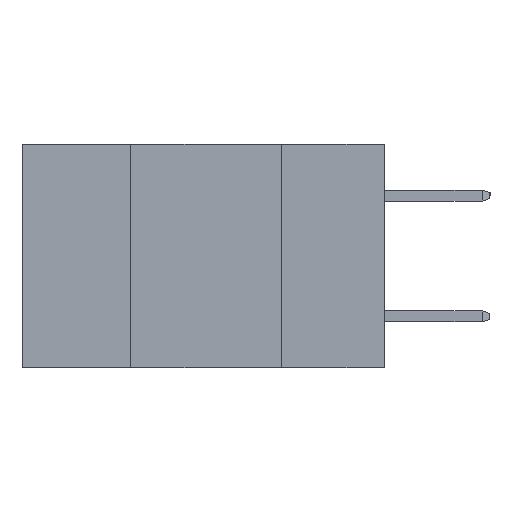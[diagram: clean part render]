
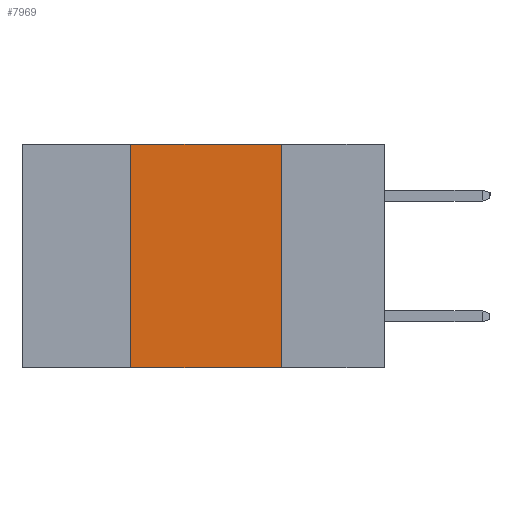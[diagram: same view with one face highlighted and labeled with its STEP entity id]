
A CAD part, left-side view. The second image highlights one B-rep face of the part: STEP entity #7969.
In plain terms, the highlighted planar face has unit normal (-1, 0, 0).
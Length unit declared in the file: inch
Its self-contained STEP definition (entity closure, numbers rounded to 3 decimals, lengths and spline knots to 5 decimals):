
#943 = DIRECTION ( 'NONE',  ( 0., 0., 1. ) ) ;
#1588 = VERTEX_POINT ( 'NONE', #14221 ) ;
#1596 = CARTESIAN_POINT ( 'NONE',  ( 0., 0.6, 0. ) ) ;
#1762 = PLANE ( 'NONE',  #10944 ) ;
#1893 = VECTOR ( 'NONE', #6723, 39.37008 ) ;
#2411 = VECTOR ( 'NONE', #6153, 39.37008 ) ;
#2767 = EDGE_LOOP ( 'NONE', ( #6430, #9768, #9889, #12947 ) ) ;
#2978 = VERTEX_POINT ( 'NONE', #11279 ) ;
#3924 = DIRECTION ( 'NONE',  ( 1., 0., 0. ) ) ;
#4325 = LINE ( 'NONE', #9272, #7523 ) ;
#4781 = CARTESIAN_POINT ( 'NONE',  ( 0., 0.42, -0.37 ) ) ;
#5536 = DIRECTION ( 'NONE',  ( 0., -1., 0. ) ) ;
#6153 = DIRECTION ( 'NONE',  ( 0., -1., 0. ) ) ;
#6430 = ORIENTED_EDGE ( 'NONE', *, *, #9613, .F. ) ;
#6723 = DIRECTION ( 'NONE',  ( 0., 0., -1. ) ) ;
#7523 = VECTOR ( 'NONE', #5536, 39.37008 ) ;
#7969 = ADVANCED_FACE ( 'NONE', ( #9104 ), #1762, .F. ) ;
#8082 = CARTESIAN_POINT ( 'NONE',  ( 0., 0.17, -0.37 ) ) ;
#8877 = DIRECTION ( 'NONE',  ( 0., 0., -1. ) ) ;
#9104 = FACE_OUTER_BOUND ( 'NONE', #2767, .T. ) ;
#9272 = CARTESIAN_POINT ( 'NONE',  ( 0., 0.6, -0.37 ) ) ;
#9613 = EDGE_CURVE ( 'NONE', #2978, #11520, #14114, .T. ) ;
#9633 = EDGE_CURVE ( 'NONE', #1588, #2978, #15714, .T. ) ;
#9768 = ORIENTED_EDGE ( 'NONE', *, *, #9633, .F. ) ;
#9889 = ORIENTED_EDGE ( 'NONE', *, *, #10138, .F. ) ;
#10138 = EDGE_CURVE ( 'NONE', #13470, #1588, #10851, .T. ) ;
#10720 = CARTESIAN_POINT ( 'NONE',  ( 0., 0.17, -0.37 ) ) ;
#10851 = LINE ( 'NONE', #4781, #11012 ) ;
#10944 = AXIS2_PLACEMENT_3D ( 'NONE', #1596, #3924, #8877 ) ;
#11012 = VECTOR ( 'NONE', #943, 39.37008 ) ;
#11279 = CARTESIAN_POINT ( 'NONE',  ( 0., 0.17, 0. ) ) ;
#11343 = CARTESIAN_POINT ( 'NONE',  ( 0., 0.42, -0.37 ) ) ;
#11520 = VERTEX_POINT ( 'NONE', #8082 ) ;
#11809 = EDGE_CURVE ( 'NONE', #13470, #11520, #4325, .T. ) ;
#12012 = CARTESIAN_POINT ( 'NONE',  ( 0., 0.6, 0. ) ) ;
#12947 = ORIENTED_EDGE ( 'NONE', *, *, #11809, .T. ) ;
#13470 = VERTEX_POINT ( 'NONE', #11343 ) ;
#14114 = LINE ( 'NONE', #10720, #1893 ) ;
#14221 = CARTESIAN_POINT ( 'NONE',  ( 0., 0.42, 0. ) ) ;
#15714 = LINE ( 'NONE', #12012, #2411 ) ;
